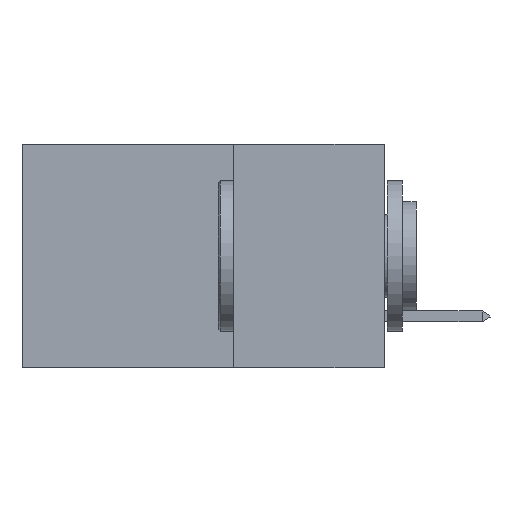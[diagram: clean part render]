
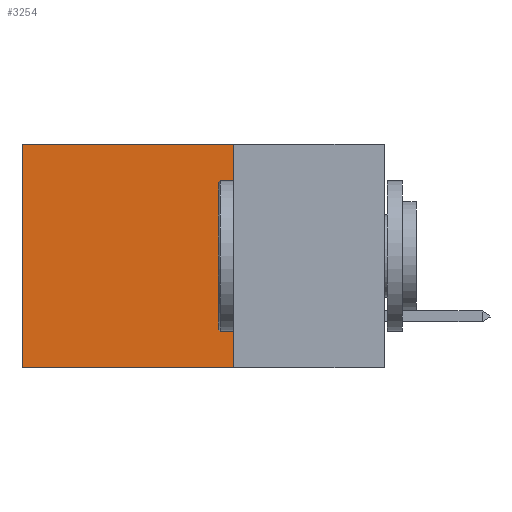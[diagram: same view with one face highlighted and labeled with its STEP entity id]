
A CAD part, left-side view. The second image highlights one B-rep face of the part: STEP entity #3254.
In plain terms, the highlighted planar face has unit normal (-1, 0, 0).
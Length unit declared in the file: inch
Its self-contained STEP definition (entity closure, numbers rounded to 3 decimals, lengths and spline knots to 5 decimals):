
#967 = CARTESIAN_POINT ( 'NONE',  ( 0.2875, 0.6, -0.37 ) ) ;
#1438 = VECTOR ( 'NONE', #4791, 39.37008 ) ;
#1828 = DIRECTION ( 'NONE',  ( 1., 0., 0. ) ) ;
#1914 = EDGE_CURVE ( 'NONE', #3887, #3836, #4688, .T. ) ;
#2165 = FACE_OUTER_BOUND ( 'NONE', #11105, .T. ) ;
#2666 = VECTOR ( 'NONE', #13036, 39.37008 ) ;
#3104 = CARTESIAN_POINT ( 'NONE',  ( 0.2875, 0.25, 0. ) ) ;
#3254 = ADVANCED_FACE ( 'NONE', ( #2165 ), #8203, .F. ) ;
#3836 = VERTEX_POINT ( 'NONE', #967 ) ;
#3887 = VERTEX_POINT ( 'NONE', #10635 ) ;
#4093 = EDGE_CURVE ( 'NONE', #6746, #6453, #4652, .T. ) ;
#4296 = ORIENTED_EDGE ( 'NONE', *, *, #13158, .T. ) ;
#4562 = LINE ( 'NONE', #6562, #10541 ) ;
#4652 = LINE ( 'NONE', #9122, #1438 ) ;
#4688 = LINE ( 'NONE', #11912, #2666 ) ;
#4791 = DIRECTION ( 'NONE',  ( 0., 0., -1. ) ) ;
#4949 = ORIENTED_EDGE ( 'NONE', *, *, #1914, .T. ) ;
#5200 = ORIENTED_EDGE ( 'NONE', *, *, #4093, .F. ) ;
#6453 = VERTEX_POINT ( 'NONE', #13778 ) ;
#6562 = CARTESIAN_POINT ( 'NONE',  ( 0.2875, 0.25, -0.37 ) ) ;
#6746 = VERTEX_POINT ( 'NONE', #10233 ) ;
#7078 = EDGE_CURVE ( 'NONE', #6453, #3836, #4562, .T. ) ;
#8203 = PLANE ( 'NONE',  #11227 ) ;
#8871 = DIRECTION ( 'NONE',  ( 0., 1., 0. ) ) ;
#9122 = CARTESIAN_POINT ( 'NONE',  ( 0.2875, 0.25, 0. ) ) ;
#10233 = CARTESIAN_POINT ( 'NONE',  ( 0.2875, 0.25, 0. ) ) ;
#10445 = DIRECTION ( 'NONE',  ( 0., 0., -1. ) ) ;
#10504 = LINE ( 'NONE', #12044, #12671 ) ;
#10518 = DIRECTION ( 'NONE',  ( 0., 1., 0. ) ) ;
#10541 = VECTOR ( 'NONE', #10518, 39.37008 ) ;
#10635 = CARTESIAN_POINT ( 'NONE',  ( 0.2875, 0.6, 0. ) ) ;
#11105 = EDGE_LOOP ( 'NONE', ( #4949, #13128, #5200, #4296 ) ) ;
#11227 = AXIS2_PLACEMENT_3D ( 'NONE', #3104, #1828, #10445 ) ;
#11912 = CARTESIAN_POINT ( 'NONE',  ( 0.2875, 0.6, 0. ) ) ;
#12044 = CARTESIAN_POINT ( 'NONE',  ( 0.2875, 0.25, 0. ) ) ;
#12671 = VECTOR ( 'NONE', #8871, 39.37008 ) ;
#13036 = DIRECTION ( 'NONE',  ( 0., 0., -1. ) ) ;
#13128 = ORIENTED_EDGE ( 'NONE', *, *, #7078, .F. ) ;
#13158 = EDGE_CURVE ( 'NONE', #6746, #3887, #10504, .T. ) ;
#13778 = CARTESIAN_POINT ( 'NONE',  ( 0.2875, 0.25, -0.37 ) ) ;
